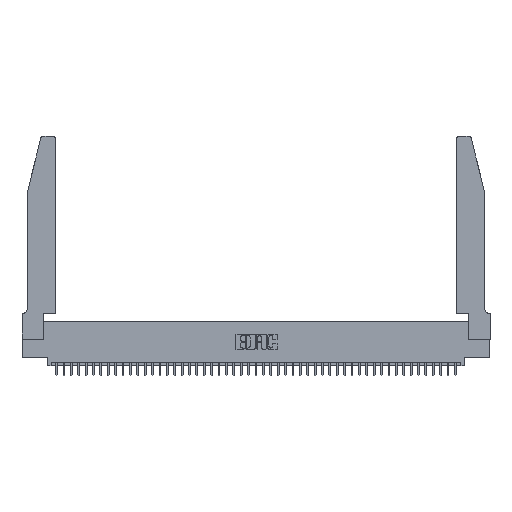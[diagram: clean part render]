
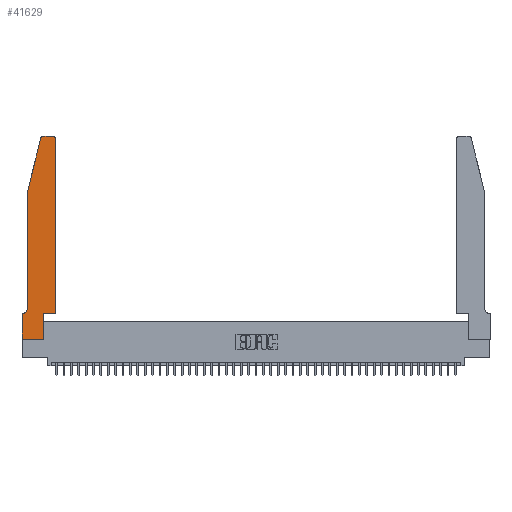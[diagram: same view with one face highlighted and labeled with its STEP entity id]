
A CAD part, top view. The second image highlights one B-rep face of the part: STEP entity #41629.
In plain terms, the highlighted planar face has unit normal (0, 0, 1).
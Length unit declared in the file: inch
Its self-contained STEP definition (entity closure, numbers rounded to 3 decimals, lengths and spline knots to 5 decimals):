
#123 = CARTESIAN_POINT ( 'NONE',  ( 0.4505, 2.72, 0.37 ) ) ;
#895 = EDGE_CURVE ( 'NONE', #17656, #28727, #42198, .T. ) ;
#1166 = DIRECTION ( 'NONE',  ( 0., 0., 1. ) ) ;
#1196 = VERTEX_POINT ( 'NONE', #32279 ) ;
#1408 = DIRECTION ( 'NONE',  ( 0., -1., 0. ) ) ;
#1473 = VERTEX_POINT ( 'NONE', #29925 ) ;
#1561 = VERTEX_POINT ( 'NONE', #8914 ) ;
#2185 = CARTESIAN_POINT ( 'NONE',  ( 0., 0.35, 0.37 ) ) ;
#2301 = VECTOR ( 'NONE', #36933, 39.37008 ) ;
#2446 = DIRECTION ( 'NONE',  ( 0., 1., 0. ) ) ;
#2475 = VECTOR ( 'NONE', #41945, 39.37008 ) ;
#2767 = CARTESIAN_POINT ( 'NONE',  ( 0.284, 2.75, 0.37 ) ) ;
#2804 = AXIS2_PLACEMENT_3D ( 'NONE', #18677, #43541, #22246 ) ;
#3473 = VECTOR ( 'NONE', #32446, 39.37008 ) ;
#3845 = CARTESIAN_POINT ( 'NONE',  ( 0.0055, 0.42, 0.37 ) ) ;
#4501 = VECTOR ( 'NONE', #1408, 39.37008 ) ;
#6406 = DIRECTION ( 'NONE',  ( 1., 0., 0. ) ) ;
#7491 = DIRECTION ( 'NONE',  ( -1., 0., 0. ) ) ;
#7819 = ORIENTED_EDGE ( 'NONE', *, *, #43699, .T. ) ;
#7827 = AXIS2_PLACEMENT_3D ( 'NONE', #22749, #1166, #26329 ) ;
#8914 = CARTESIAN_POINT ( 'NONE',  ( 0.0755, 2., 0.37 ) ) ;
#8982 = ORIENTED_EDGE ( 'NONE', *, *, #32632, .T. ) ;
#9115 = LINE ( 'NONE', #14803, #44857 ) ;
#9290 = DIRECTION ( 'NONE',  ( 0., 0., 1. ) ) ;
#9674 = EDGE_CURVE ( 'NONE', #1196, #17656, #9115, .T. ) ;
#9804 = EDGE_CURVE ( 'NONE', #44546, #12462, #21491, .T. ) ;
#9998 = VERTEX_POINT ( 'NONE', #24151 ) ;
#10986 = LINE ( 'NONE', #17028, #2475 ) ;
#12027 = ORIENTED_EDGE ( 'NONE', *, *, #9674, .T. ) ;
#12247 = CARTESIAN_POINT ( 'NONE',  ( 0.4505, 0.35, 0.37 ) ) ;
#12462 = VERTEX_POINT ( 'NONE', #2185 ) ;
#12789 = CIRCLE ( 'NONE', #2804, 0.03 ) ;
#13125 = LINE ( 'NONE', #42992, #3473 ) ;
#14803 = CARTESIAN_POINT ( 'NONE',  ( 0.2605, 2.75, 0.37 ) ) ;
#16017 = VECTOR ( 'NONE', #22139, 39.37008 ) ;
#16358 = EDGE_CURVE ( 'NONE', #12462, #9998, #17576, .T. ) ;
#16852 = EDGE_CURVE ( 'NONE', #1561, #38578, #43683, .T. ) ;
#17028 = CARTESIAN_POINT ( 'NONE',  ( 0., 0., 0.37 ) ) ;
#17576 = LINE ( 'NONE', #27410, #34308 ) ;
#17656 = VERTEX_POINT ( 'NONE', #2767 ) ;
#18422 = DIRECTION ( 'NONE',  ( -1., 0., 0. ) ) ;
#18574 = CARTESIAN_POINT ( 'NONE',  ( 0.0755, 2., 0.37 ) ) ;
#18677 = CARTESIAN_POINT ( 'NONE',  ( 0.4205, 2.72, 0.37 ) ) ;
#18880 = ORIENTED_EDGE ( 'NONE', *, *, #25519, .T. ) ;
#19182 = CARTESIAN_POINT ( 'NONE',  ( 0.0755, 0.35, 0.37 ) ) ;
#19289 = VECTOR ( 'NONE', #6406, 39.37008 ) ;
#19414 = CARTESIAN_POINT ( 'NONE',  ( 0.0755, 2., 0.37 ) ) ;
#20448 = LINE ( 'NONE', #31339, #19289 ) ;
#20863 = CARTESIAN_POINT ( 'NONE',  ( 0.25487, 2.72718, 0.37 ) ) ;
#20977 = CIRCLE ( 'NONE', #28944, 0.07 ) ;
#21088 = ORIENTED_EDGE ( 'NONE', *, *, #25714, .T. ) ;
#21491 = LINE ( 'NONE', #19182, #2301 ) ;
#22139 = DIRECTION ( 'NONE',  ( -0.239, -0.971, 0. ) ) ;
#22246 = DIRECTION ( 'NONE',  ( 1., 0., 0. ) ) ;
#22749 = CARTESIAN_POINT ( 'NONE',  ( 0., 0.35, 0.37 ) ) ;
#23303 = VERTEX_POINT ( 'NONE', #43924 ) ;
#24151 = CARTESIAN_POINT ( 'NONE',  ( 0., 0., 0.37 ) ) ;
#25285 = LINE ( 'NONE', #45299, #41966 ) ;
#25519 = EDGE_CURVE ( 'NONE', #1473, #44115, #20448, .T. ) ;
#25714 = EDGE_CURVE ( 'NONE', #38578, #44546, #20977, .T. ) ;
#26329 = DIRECTION ( 'NONE',  ( 1., 0., 0. ) ) ;
#27410 = CARTESIAN_POINT ( 'NONE',  ( 0., 0., 0.37 ) ) ;
#27655 = VERTEX_POINT ( 'NONE', #123 ) ;
#28727 = VERTEX_POINT ( 'NONE', #20863 ) ;
#28944 = AXIS2_PLACEMENT_3D ( 'NONE', #3845, #28981, #7491 ) ;
#28981 = DIRECTION ( 'NONE',  ( 0., 0., -1. ) ) ;
#29925 = CARTESIAN_POINT ( 'NONE',  ( 0.2865, 0.35, 0.37 ) ) ;
#30747 = CARTESIAN_POINT ( 'NONE',  ( 0.284, 2.72, 0.37 ) ) ;
#31319 = ORIENTED_EDGE ( 'NONE', *, *, #41457, .T. ) ;
#31339 = CARTESIAN_POINT ( 'NONE',  ( 0.4505, 0.35, 0.37 ) ) ;
#32279 = CARTESIAN_POINT ( 'NONE',  ( 0.4205, 2.75, 0.37 ) ) ;
#32446 = DIRECTION ( 'NONE',  ( 0., 1., 0. ) ) ;
#32632 = EDGE_CURVE ( 'NONE', #9998, #23303, #10986, .T. ) ;
#32646 = FACE_OUTER_BOUND ( 'NONE', #36147, .T. ) ;
#33208 = ORIENTED_EDGE ( 'NONE', *, *, #38947, .T. ) ;
#33519 = ORIENTED_EDGE ( 'NONE', *, *, #895, .T. ) ;
#33888 = LINE ( 'NONE', #18574, #16017 ) ;
#34308 = VECTOR ( 'NONE', #34584, 39.37008 ) ;
#34330 = DIRECTION ( 'NONE',  ( 1., 0., 0. ) ) ;
#34584 = DIRECTION ( 'NONE',  ( 0., -1., 0. ) ) ;
#35811 = CARTESIAN_POINT ( 'NONE',  ( 0.0055, 0.35, 0.37 ) ) ;
#35832 = ORIENTED_EDGE ( 'NONE', *, *, #16852, .T. ) ;
#36147 = EDGE_LOOP ( 'NONE', ( #12027, #33519, #44473, #35832, #21088, #37113, #42298, #8982, #31319, #18880, #7819, #33208 ) ) ;
#36930 = PLANE ( 'NONE',  #7827 ) ;
#36933 = DIRECTION ( 'NONE',  ( -1., 0., 0. ) ) ;
#37113 = ORIENTED_EDGE ( 'NONE', *, *, #9804, .T. ) ;
#37370 = CARTESIAN_POINT ( 'NONE',  ( 0.0755, 0.42, 0.37 ) ) ;
#38578 = VERTEX_POINT ( 'NONE', #37370 ) ;
#38947 = EDGE_CURVE ( 'NONE', #27655, #1196, #12789, .T. ) ;
#40281 = EDGE_CURVE ( 'NONE', #28727, #1561, #33888, .T. ) ;
#41457 = EDGE_CURVE ( 'NONE', #23303, #1473, #13125, .T. ) ;
#41629 = ADVANCED_FACE ( 'NONE', ( #32646 ), #36930, .T. ) ;
#41945 = DIRECTION ( 'NONE',  ( 1., 0., 0. ) ) ;
#41966 = VECTOR ( 'NONE', #2446, 39.37008 ) ;
#42198 = CIRCLE ( 'NONE', #45002, 0.03 ) ;
#42298 = ORIENTED_EDGE ( 'NONE', *, *, #16358, .T. ) ;
#42992 = CARTESIAN_POINT ( 'NONE',  ( 0.2865, 0.35, 0.37 ) ) ;
#43541 = DIRECTION ( 'NONE',  ( 0., 0., 1. ) ) ;
#43683 = LINE ( 'NONE', #19414, #4501 ) ;
#43699 = EDGE_CURVE ( 'NONE', #44115, #27655, #25285, .T. ) ;
#43924 = CARTESIAN_POINT ( 'NONE',  ( 0.2865, 0., 0.37 ) ) ;
#44115 = VERTEX_POINT ( 'NONE', #12247 ) ;
#44473 = ORIENTED_EDGE ( 'NONE', *, *, #40281, .T. ) ;
#44546 = VERTEX_POINT ( 'NONE', #35811 ) ;
#44857 = VECTOR ( 'NONE', #18422, 39.37008 ) ;
#45002 = AXIS2_PLACEMENT_3D ( 'NONE', #30747, #9290, #34330 ) ;
#45299 = CARTESIAN_POINT ( 'NONE',  ( 0.4505, 0.35, 0.37 ) ) ;
